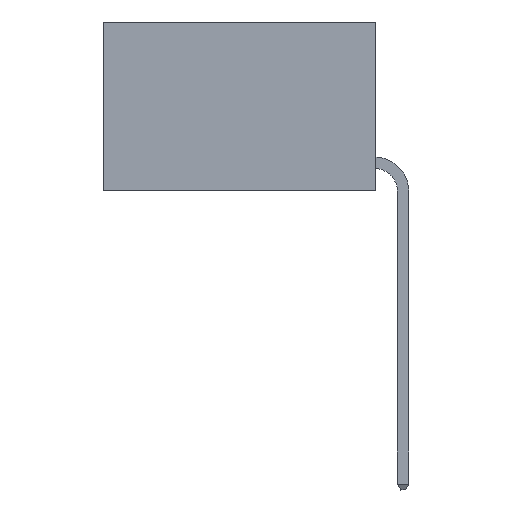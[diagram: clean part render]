
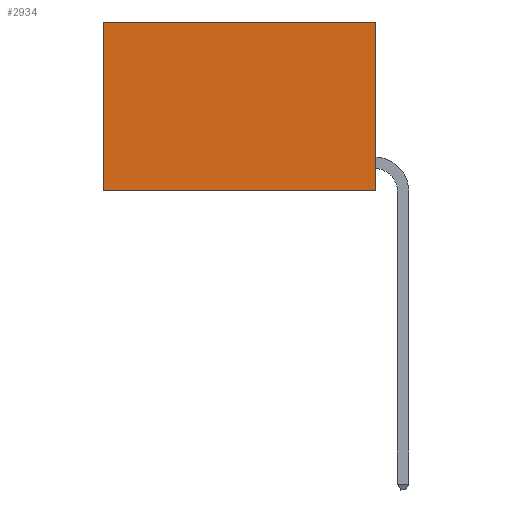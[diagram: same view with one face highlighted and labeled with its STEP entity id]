
A CAD part, left-side view. The second image highlights one B-rep face of the part: STEP entity #2934.
In plain terms, the highlighted planar face has unit normal (-1, 0, 0).
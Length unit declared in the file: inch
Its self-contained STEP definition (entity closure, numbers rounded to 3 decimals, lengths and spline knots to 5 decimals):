
#1082 = DIRECTION ( 'NONE',  ( 1., 0., 0. ) ) ;
#1481 = CARTESIAN_POINT ( 'NONE',  ( 0.2625, 0., 0. ) ) ;
#1824 = LINE ( 'NONE', #1481, #14341 ) ;
#2051 = EDGE_CURVE ( 'NONE', #15581, #7454, #11265, .T. ) ;
#2418 = LINE ( 'NONE', #10347, #14398 ) ;
#2632 = CARTESIAN_POINT ( 'NONE',  ( 0.2625, 0.6, 0. ) ) ;
#2934 = ADVANCED_FACE ( 'NONE', ( #14539 ), #17332, .F. ) ;
#3041 = ORIENTED_EDGE ( 'NONE', *, *, #2051, .F. ) ;
#3194 = DIRECTION ( 'NONE',  ( 0., 1., 0. ) ) ;
#3585 = CARTESIAN_POINT ( 'NONE',  ( 0.2625, 0.6, -0.37 ) ) ;
#4149 = CARTESIAN_POINT ( 'NONE',  ( 0.2625, 0.6, 0. ) ) ;
#4886 = AXIS2_PLACEMENT_3D ( 'NONE', #17786, #1082, #13541 ) ;
#7454 = VERTEX_POINT ( 'NONE', #14285 ) ;
#7562 = EDGE_CURVE ( 'NONE', #15581, #16267, #1824, .T. ) ;
#10347 = CARTESIAN_POINT ( 'NONE',  ( 0.2625, 0., -0.37 ) ) ;
#10483 = EDGE_CURVE ( 'NONE', #16267, #10732, #17566, .T. ) ;
#10732 = VERTEX_POINT ( 'NONE', #3585 ) ;
#11265 = LINE ( 'NONE', #11556, #19776 ) ;
#11556 = CARTESIAN_POINT ( 'NONE',  ( 0.2625, 0., 0. ) ) ;
#11934 = CARTESIAN_POINT ( 'NONE',  ( 0.2625, 0., 0. ) ) ;
#11951 = DIRECTION ( 'NONE',  ( 0., 1., 0. ) ) ;
#12524 = ORIENTED_EDGE ( 'NONE', *, *, #10483, .T. ) ;
#13541 = DIRECTION ( 'NONE',  ( 0., 0., -1. ) ) ;
#14285 = CARTESIAN_POINT ( 'NONE',  ( 0.2625, 0., -0.37 ) ) ;
#14341 = VECTOR ( 'NONE', #3194, 39.37008 ) ;
#14398 = VECTOR ( 'NONE', #11951, 39.37008 ) ;
#14539 = FACE_OUTER_BOUND ( 'NONE', #20385, .T. ) ;
#15284 = DIRECTION ( 'NONE',  ( 0., 0., -1. ) ) ;
#15581 = VERTEX_POINT ( 'NONE', #11934 ) ;
#15638 = DIRECTION ( 'NONE',  ( 0., 0., -1. ) ) ;
#16267 = VERTEX_POINT ( 'NONE', #4149 ) ;
#16294 = ORIENTED_EDGE ( 'NONE', *, *, #18010, .F. ) ;
#16603 = VECTOR ( 'NONE', #15638, 39.37008 ) ;
#16629 = ORIENTED_EDGE ( 'NONE', *, *, #7562, .T. ) ;
#17332 = PLANE ( 'NONE',  #4886 ) ;
#17566 = LINE ( 'NONE', #2632, #16603 ) ;
#17786 = CARTESIAN_POINT ( 'NONE',  ( 0.2625, 0., 0. ) ) ;
#18010 = EDGE_CURVE ( 'NONE', #7454, #10732, #2418, .T. ) ;
#19776 = VECTOR ( 'NONE', #15284, 39.37008 ) ;
#20385 = EDGE_LOOP ( 'NONE', ( #12524, #16294, #3041, #16629 ) ) ;
